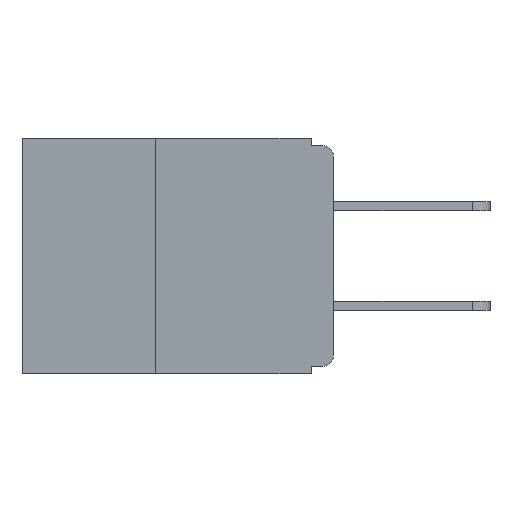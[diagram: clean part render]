
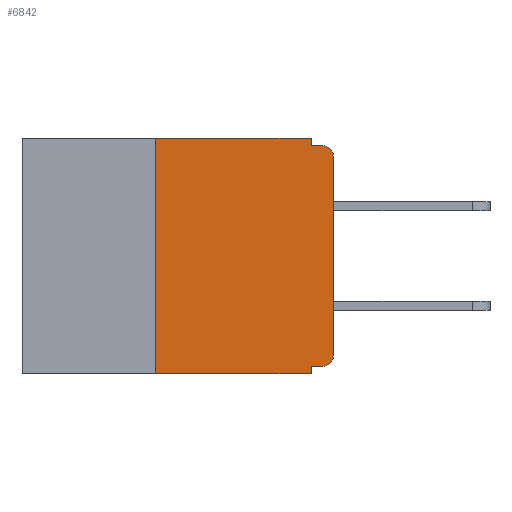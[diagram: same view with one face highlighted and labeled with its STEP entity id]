
A CAD part, left-side view. The second image highlights one B-rep face of the part: STEP entity #6842.
In plain terms, the highlighted planar face has unit normal (-1, 0, 0).
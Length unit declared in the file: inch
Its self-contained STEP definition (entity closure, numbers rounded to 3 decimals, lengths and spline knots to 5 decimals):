
#112 = DIRECTION ( 'NONE',  ( 0., 0., -1. ) ) ;
#122 = ORIENTED_EDGE ( 'NONE', *, *, #4369, .F. ) ;
#254 = VERTEX_POINT ( 'NONE', #4184 ) ;
#268 = ORIENTED_EDGE ( 'NONE', *, *, #13794, .F. ) ;
#284 = ORIENTED_EDGE ( 'NONE', *, *, #12856, .F. ) ;
#311 = DIRECTION ( 'NONE',  ( 0., -1., 0. ) ) ;
#333 = ORIENTED_EDGE ( 'NONE', *, *, #782, .F. ) ;
#523 = VERTEX_POINT ( 'NONE', #14588 ) ;
#687 = CARTESIAN_POINT ( 'NONE',  ( 0., 0.25, -0.33 ) ) ;
#782 = EDGE_CURVE ( 'NONE', #7061, #523, #5950, .T. ) ;
#887 = VECTOR ( 'NONE', #5251, 39.37008 ) ;
#902 = AXIS2_PLACEMENT_3D ( 'NONE', #13683, #6861, #112 ) ;
#939 = LINE ( 'NONE', #8850, #3559 ) ;
#1467 = CARTESIAN_POINT ( 'NONE',  ( 0., 0.015, -0.025 ) ) ;
#1630 = VERTEX_POINT ( 'NONE', #13753 ) ;
#1778 = FACE_OUTER_BOUND ( 'NONE', #3804, .T. ) ;
#2586 = DIRECTION ( 'NONE',  ( 0., 0., -1. ) ) ;
#2606 = VECTOR ( 'NONE', #11122, 39.37008 ) ;
#2636 = CARTESIAN_POINT ( 'NONE',  ( 0., 0.031, 0. ) ) ;
#2778 = VERTEX_POINT ( 'NONE', #7793 ) ;
#3233 = DIRECTION ( 'NONE',  ( 0., 0., 1. ) ) ;
#3330 = VECTOR ( 'NONE', #3233, 39.37008 ) ;
#3363 = CARTESIAN_POINT ( 'NONE',  ( 0., 0., 0. ) ) ;
#3559 = VECTOR ( 'NONE', #7743, 39.37008 ) ;
#3572 = ORIENTED_EDGE ( 'NONE', *, *, #7851, .T. ) ;
#3804 = EDGE_LOOP ( 'NONE', ( #3572, #14494, #13520, #268, #6872, #284, #9011, #333, #122, #5184 ) ) ;
#4126 = VERTEX_POINT ( 'NONE', #6713 ) ;
#4184 = CARTESIAN_POINT ( 'NONE',  ( 0., 0.031, -0.01 ) ) ;
#4243 = LINE ( 'NONE', #687, #887 ) ;
#4369 = EDGE_CURVE ( 'NONE', #4126, #7061, #13177, .T. ) ;
#4512 = VECTOR ( 'NONE', #13608, 39.37008 ) ;
#4849 = EDGE_CURVE ( 'NONE', #254, #2778, #12798, .T. ) ;
#4985 = VERTEX_POINT ( 'NONE', #13432 ) ;
#5025 = CARTESIAN_POINT ( 'NONE',  ( 0., 0., -0.32 ) ) ;
#5184 = ORIENTED_EDGE ( 'NONE', *, *, #13148, .T. ) ;
#5251 = DIRECTION ( 'NONE',  ( 0., 0., 1. ) ) ;
#5489 = CARTESIAN_POINT ( 'NONE',  ( 0., 0., -0.025 ) ) ;
#5950 = LINE ( 'NONE', #14170, #2606 ) ;
#6299 = LINE ( 'NONE', #3363, #3330 ) ;
#6713 = CARTESIAN_POINT ( 'NONE',  ( 0., 0.015, -0.32 ) ) ;
#6806 = VECTOR ( 'NONE', #12809, 39.37008 ) ;
#6842 = ADVANCED_FACE ( 'NONE', ( #1778 ), #13075, .F. ) ;
#6861 = DIRECTION ( 'NONE',  ( -1., 0., 0. ) ) ;
#6872 = ORIENTED_EDGE ( 'NONE', *, *, #12859, .F. ) ;
#7061 = VERTEX_POINT ( 'NONE', #10854 ) ;
#7212 = CIRCLE ( 'NONE', #14410, 0.015 ) ;
#7743 = DIRECTION ( 'NONE',  ( 0., -1., 0. ) ) ;
#7793 = CARTESIAN_POINT ( 'NONE',  ( 0., 0.015, -0.01 ) ) ;
#7851 = EDGE_CURVE ( 'NONE', #4985, #9097, #6299, .T. ) ;
#8220 = VECTOR ( 'NONE', #10804, 39.37008 ) ;
#8850 = CARTESIAN_POINT ( 'NONE',  ( 0., 0.437, -0.33 ) ) ;
#9011 = ORIENTED_EDGE ( 'NONE', *, *, #10902, .T. ) ;
#9033 = AXIS2_PLACEMENT_3D ( 'NONE', #12984, #12875, #12796 ) ;
#9097 = VERTEX_POINT ( 'NONE', #5489 ) ;
#9250 = DIRECTION ( 'NONE',  ( -1., 0., 0. ) ) ;
#9696 = CARTESIAN_POINT ( 'NONE',  ( 0., 0.25, -0.33 ) ) ;
#9700 = VECTOR ( 'NONE', #311, 39.37008 ) ;
#10144 = CARTESIAN_POINT ( 'NONE',  ( 0., 0.031, 0. ) ) ;
#10804 = DIRECTION ( 'NONE',  ( 0., -1., 0. ) ) ;
#10854 = CARTESIAN_POINT ( 'NONE',  ( 0., 0.031, -0.32 ) ) ;
#10902 = EDGE_CURVE ( 'NONE', #12233, #523, #939, .T. ) ;
#11122 = DIRECTION ( 'NONE',  ( 0., 0., -1. ) ) ;
#11389 = CARTESIAN_POINT ( 'NONE',  ( 0., 0., -0.01 ) ) ;
#11868 = VERTEX_POINT ( 'NONE', #10144 ) ;
#11997 = EDGE_CURVE ( 'NONE', #9097, #2778, #7212, .T. ) ;
#12233 = VERTEX_POINT ( 'NONE', #9696 ) ;
#12507 = LINE ( 'NONE', #2636, #6806 ) ;
#12716 = CIRCLE ( 'NONE', #902, 0.015 ) ;
#12796 = DIRECTION ( 'NONE',  ( 0., 0., -1. ) ) ;
#12798 = LINE ( 'NONE', #11389, #9700 ) ;
#12809 = DIRECTION ( 'NONE',  ( 0., 0., -1. ) ) ;
#12856 = EDGE_CURVE ( 'NONE', #12233, #1630, #4243, .T. ) ;
#12859 = EDGE_CURVE ( 'NONE', #1630, #11868, #12898, .T. ) ;
#12875 = DIRECTION ( 'NONE',  ( 1., 0., 0. ) ) ;
#12898 = LINE ( 'NONE', #13139, #8220 ) ;
#12984 = CARTESIAN_POINT ( 'NONE',  ( 0., 0.437, 0. ) ) ;
#13075 = PLANE ( 'NONE',  #9033 ) ;
#13139 = CARTESIAN_POINT ( 'NONE',  ( 0., 0.437, 0. ) ) ;
#13148 = EDGE_CURVE ( 'NONE', #4126, #4985, #12716, .T. ) ;
#13177 = LINE ( 'NONE', #5025, #4512 ) ;
#13432 = CARTESIAN_POINT ( 'NONE',  ( 0., 0., -0.305 ) ) ;
#13520 = ORIENTED_EDGE ( 'NONE', *, *, #4849, .F. ) ;
#13608 = DIRECTION ( 'NONE',  ( 0., 1., 0. ) ) ;
#13683 = CARTESIAN_POINT ( 'NONE',  ( 0., 0.015, -0.305 ) ) ;
#13753 = CARTESIAN_POINT ( 'NONE',  ( 0., 0.25, 0. ) ) ;
#13794 = EDGE_CURVE ( 'NONE', #11868, #254, #12507, .T. ) ;
#14170 = CARTESIAN_POINT ( 'NONE',  ( 0., 0.031, -0.33 ) ) ;
#14410 = AXIS2_PLACEMENT_3D ( 'NONE', #1467, #9250, #2586 ) ;
#14494 = ORIENTED_EDGE ( 'NONE', *, *, #11997, .T. ) ;
#14588 = CARTESIAN_POINT ( 'NONE',  ( 0., 0.031, -0.33 ) ) ;
